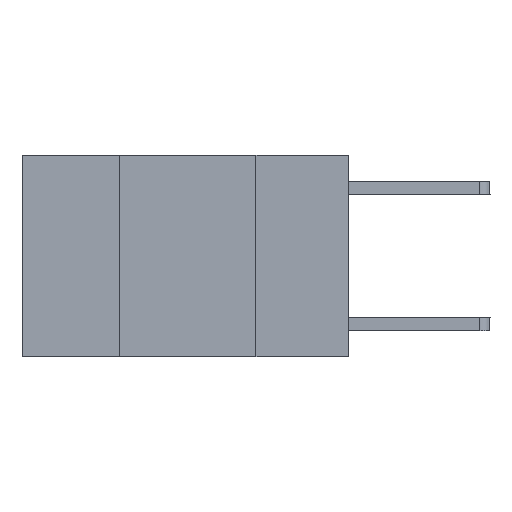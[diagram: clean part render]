
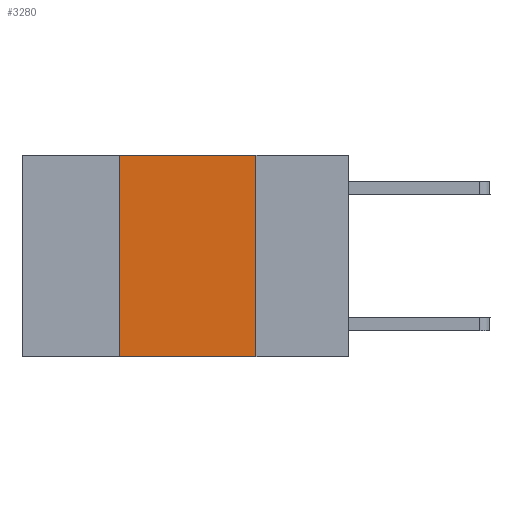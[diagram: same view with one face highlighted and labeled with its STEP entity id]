
A CAD part, left-side view. The second image highlights one B-rep face of the part: STEP entity #3280.
In plain terms, the highlighted planar face has unit normal (-1, 0, 0).
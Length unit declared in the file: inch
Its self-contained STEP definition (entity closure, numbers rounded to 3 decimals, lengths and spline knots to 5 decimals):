
#23 = LINE ( 'NONE', #887, #3328 ) ;
#119 = DIRECTION ( 'NONE',  ( 0., 0., 1. ) ) ;
#545 = DIRECTION ( 'NONE',  ( 0., -1., 0. ) ) ;
#887 = CARTESIAN_POINT ( 'NONE',  ( 0., 0.17, 0. ) ) ;
#901 = ORIENTED_EDGE ( 'NONE', *, *, #4458, .T. ) ;
#1686 = DIRECTION ( 'NONE',  ( 0., -1., 0. ) ) ;
#2993 = CARTESIAN_POINT ( 'NONE',  ( 0., 0.6, 0. ) ) ;
#3092 = CARTESIAN_POINT ( 'NONE',  ( 0., 0.17, -0.37 ) ) ;
#3143 = DIRECTION ( 'NONE',  ( 1., 0., 0. ) ) ;
#3280 = ADVANCED_FACE ( 'NONE', ( #8323 ), #11027, .F. ) ;
#3328 = VECTOR ( 'NONE', #5961, 39.37008 ) ;
#3563 = EDGE_CURVE ( 'NONE', #6095, #11064, #6472, .T. ) ;
#3978 = CARTESIAN_POINT ( 'NONE',  ( 0., 0.17, 0. ) ) ;
#4458 = EDGE_CURVE ( 'NONE', #6095, #4753, #9619, .T. ) ;
#4560 = CARTESIAN_POINT ( 'NONE',  ( 0., 0.42, 0. ) ) ;
#4753 = VERTEX_POINT ( 'NONE', #3092 ) ;
#5663 = VECTOR ( 'NONE', #119, 39.37008 ) ;
#5778 = DIRECTION ( 'NONE',  ( 0., 0., -1. ) ) ;
#5836 = VECTOR ( 'NONE', #545, 39.37008 ) ;
#5961 = DIRECTION ( 'NONE',  ( 0., 0., -1. ) ) ;
#6095 = VERTEX_POINT ( 'NONE', #9220 ) ;
#6293 = EDGE_CURVE ( 'NONE', #7291, #4753, #23, .T. ) ;
#6472 = LINE ( 'NONE', #7968, #5663 ) ;
#6597 = CARTESIAN_POINT ( 'NONE',  ( 0., 0.6, 0. ) ) ;
#6974 = VECTOR ( 'NONE', #1686, 39.37008 ) ;
#7291 = VERTEX_POINT ( 'NONE', #3978 ) ;
#7686 = ORIENTED_EDGE ( 'NONE', *, *, #6293, .F. ) ;
#7968 = CARTESIAN_POINT ( 'NONE',  ( 0., 0.42, 0. ) ) ;
#8215 = AXIS2_PLACEMENT_3D ( 'NONE', #6597, #3143, #5778 ) ;
#8323 = FACE_OUTER_BOUND ( 'NONE', #9666, .T. ) ;
#9220 = CARTESIAN_POINT ( 'NONE',  ( 0., 0.42, -0.37 ) ) ;
#9368 = ORIENTED_EDGE ( 'NONE', *, *, #10006, .F. ) ;
#9619 = LINE ( 'NONE', #11208, #6974 ) ;
#9666 = EDGE_LOOP ( 'NONE', ( #7686, #9368, #10716, #901 ) ) ;
#10006 = EDGE_CURVE ( 'NONE', #11064, #7291, #10876, .T. ) ;
#10716 = ORIENTED_EDGE ( 'NONE', *, *, #3563, .F. ) ;
#10876 = LINE ( 'NONE', #2993, #5836 ) ;
#11027 = PLANE ( 'NONE',  #8215 ) ;
#11064 = VERTEX_POINT ( 'NONE', #4560 ) ;
#11208 = CARTESIAN_POINT ( 'NONE',  ( 0., 0.6, -0.37 ) ) ;
